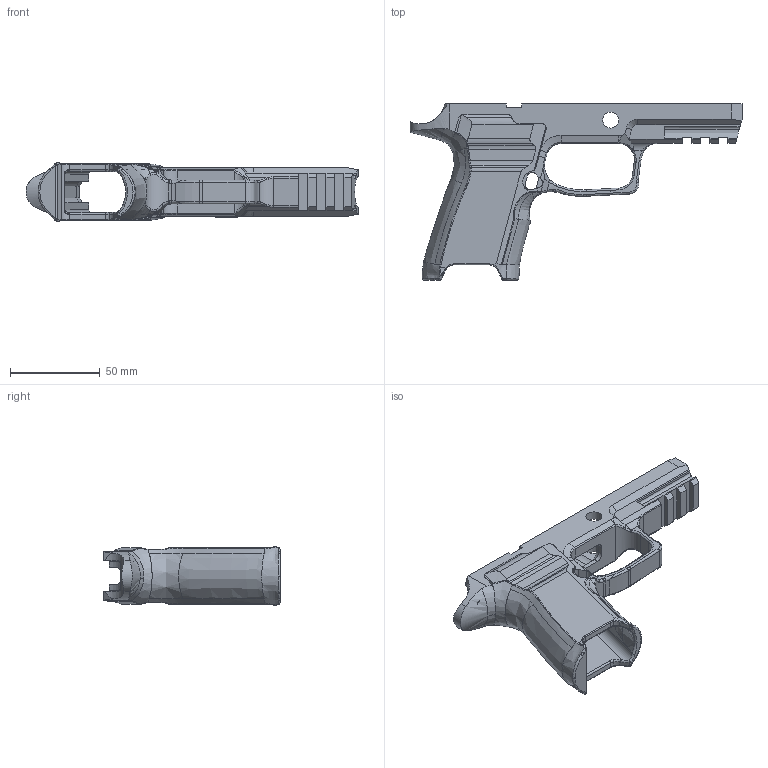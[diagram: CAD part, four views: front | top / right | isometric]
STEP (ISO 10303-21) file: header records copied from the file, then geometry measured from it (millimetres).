
FILE_DESCRIPTION(/* description */ (''),/* implementation_level */ '2;1');
FILE_NAME(/* name */ 'JP320 Compact Grip Module.step',/* time_stamp */ '2023-02-07T19:32:23-05:00',/* author */ (''),/* organization */ (''),/* preprocessor_version */ 'ST-DEVELOPER v19.2',/* originating_system */ 'Autodesk Translation Framework v11.17.0.187',/* authorisation */ '');
FILE_SCHEMA (('AUTOMOTIVE_DESIGN { 1 0 10303 214 3 1 1 }'));
Products named in the file (5): JP320 Grip Module; JP320 Grip Module_1; Compact; Common Parts; FCU Plug
Assembly tree (4 placements, depth 3):
  JP320 Grip Module
    JP320 Grip Module_1
      Compact
    Common Parts
      FCU Plug
Bounding box: 184.6 x 98 x 33.01 mm (x, y, z)
Volume: 80242 mm3; surface area: 44474.4 mm2
Topology: 2 solids, 2 shells, 548 faces, 1601 edges, 1041 vertices
Faces by surface type: plane 206, bspline 179, cylinder 132, torus 17, cone 8, sphere 6
Full cylindrical faces by diameter (mm): 8.9 x1, 9.4 x1
Entity records: 52522 total; most frequent: CARTESIAN_POINT 38828, ORIENTED_EDGE 3186, DIRECTION 2428, EDGE_CURVE 1593, VERTEX_POINT 1041, AXIS2_PLACEMENT_3D 861, LINE 706, VECTOR 706
